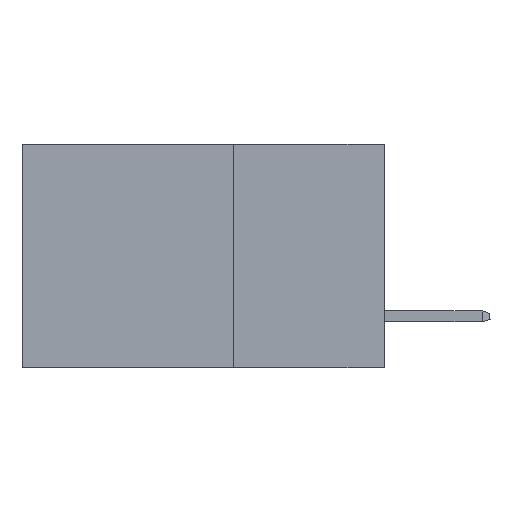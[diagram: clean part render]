
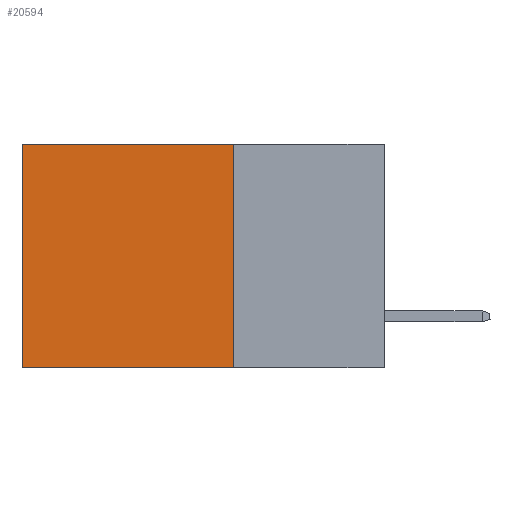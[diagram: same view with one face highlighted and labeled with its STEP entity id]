
A CAD part, left-side view. The second image highlights one B-rep face of the part: STEP entity #20594.
In plain terms, the highlighted planar face has unit normal (-1, 0, 0).
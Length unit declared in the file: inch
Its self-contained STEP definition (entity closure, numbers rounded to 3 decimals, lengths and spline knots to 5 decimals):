
#71 = VERTEX_POINT ( 'NONE', #19848 ) ;
#174 = VERTEX_POINT ( 'NONE', #17552 ) ;
#816 = EDGE_CURVE ( 'NONE', #31631, #2164, #9800, .T. ) ;
#1189 = AXIS2_PLACEMENT_3D ( 'NONE', #7733, #18225, #23699 ) ;
#2164 = VERTEX_POINT ( 'NONE', #22490 ) ;
#3074 = EDGE_CURVE ( 'NONE', #31631, #174, #6532, .T. ) ;
#3866 = ORIENTED_EDGE ( 'NONE', *, *, #3074, .F. ) ;
#4373 = ORIENTED_EDGE ( 'NONE', *, *, #9595, .F. ) ;
#6532 = LINE ( 'NONE', #22308, #13562 ) ;
#7733 = CARTESIAN_POINT ( 'NONE',  ( 0.298, 0.25, 0. ) ) ;
#8900 = LINE ( 'NONE', #21161, #28064 ) ;
#9595 = EDGE_CURVE ( 'NONE', #174, #71, #11175, .T. ) ;
#9800 = LINE ( 'NONE', #23486, #26622 ) ;
#11175 = LINE ( 'NONE', #26426, #19009 ) ;
#12649 = ORIENTED_EDGE ( 'NONE', *, *, #30687, .T. ) ;
#13562 = VECTOR ( 'NONE', #17271, 39.37008 ) ;
#14105 = DIRECTION ( 'NONE',  ( 0., 1., 0. ) ) ;
#15304 = PLANE ( 'NONE',  #1189 ) ;
#15847 = CARTESIAN_POINT ( 'NONE',  ( 0.298, 0.25, 0. ) ) ;
#17271 = DIRECTION ( 'NONE',  ( 0., 0., -1. ) ) ;
#17305 = FACE_OUTER_BOUND ( 'NONE', #20815, .T. ) ;
#17552 = CARTESIAN_POINT ( 'NONE',  ( 0.298, 0.25, -0.37 ) ) ;
#18225 = DIRECTION ( 'NONE',  ( 1., 0., 0. ) ) ;
#19009 = VECTOR ( 'NONE', #14105, 39.37008 ) ;
#19848 = CARTESIAN_POINT ( 'NONE',  ( 0.298, 0.6, -0.37 ) ) ;
#20594 = ADVANCED_FACE ( 'NONE', ( #17305 ), #15304, .F. ) ;
#20815 = EDGE_LOOP ( 'NONE', ( #12649, #4373, #3866, #26319 ) ) ;
#21161 = CARTESIAN_POINT ( 'NONE',  ( 0.298, 0.6, 0. ) ) ;
#21267 = DIRECTION ( 'NONE',  ( 0., 0., -1. ) ) ;
#21271 = DIRECTION ( 'NONE',  ( 0., 1., 0. ) ) ;
#22308 = CARTESIAN_POINT ( 'NONE',  ( 0.298, 0.25, 0. ) ) ;
#22490 = CARTESIAN_POINT ( 'NONE',  ( 0.298, 0.6, 0. ) ) ;
#23486 = CARTESIAN_POINT ( 'NONE',  ( 0.298, 0.25, 0. ) ) ;
#23699 = DIRECTION ( 'NONE',  ( 0., 0., -1. ) ) ;
#26319 = ORIENTED_EDGE ( 'NONE', *, *, #816, .T. ) ;
#26426 = CARTESIAN_POINT ( 'NONE',  ( 0.298, 0.25, -0.37 ) ) ;
#26622 = VECTOR ( 'NONE', #21271, 39.37008 ) ;
#28064 = VECTOR ( 'NONE', #21267, 39.37008 ) ;
#30687 = EDGE_CURVE ( 'NONE', #2164, #71, #8900, .T. ) ;
#31631 = VERTEX_POINT ( 'NONE', #15847 ) ;
